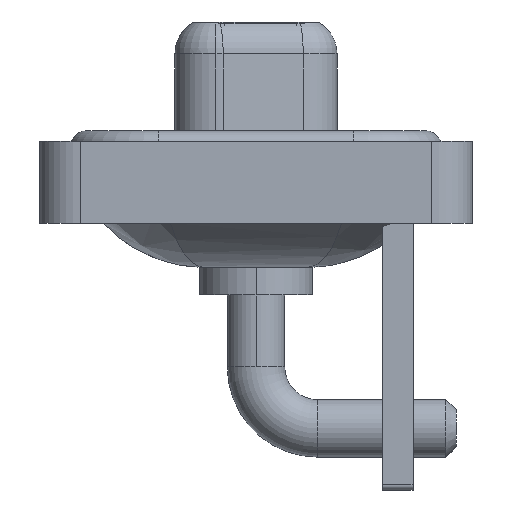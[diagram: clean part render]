
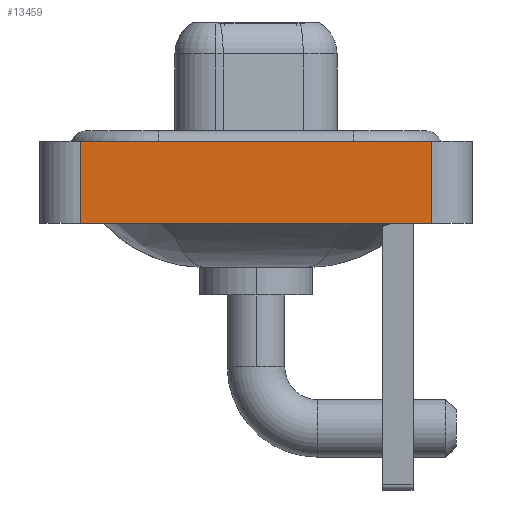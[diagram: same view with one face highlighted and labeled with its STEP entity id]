
A CAD part, left-side view. The second image highlights one B-rep face of the part: STEP entity #13459.
In plain terms, the highlighted planar face has unit normal (-1, 0, 0).
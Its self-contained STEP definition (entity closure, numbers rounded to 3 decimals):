
#3 = ORIENTED_EDGE ( 'NONE', *, *, #13370, .F. ) ;
#154 = ORIENTED_EDGE ( 'NONE', *, *, #11582, .T. ) ;
#654 = VERTEX_POINT ( 'NONE', #11953 ) ;
#843 = EDGE_LOOP ( 'NONE', ( #16155, #3, #2913, #154 ) ) ;
#848 = VERTEX_POINT ( 'NONE', #10019 ) ;
#1417 = DIRECTION ( 'NONE',  ( 0., -1., 0. ) ) ;
#1801 = VECTOR ( 'NONE', #1417, 1000. ) ;
#1831 = FACE_OUTER_BOUND ( 'NONE', #843, .T. ) ;
#2157 = CARTESIAN_POINT ( 'NONE',  ( -7.25, -8.55, 0.4 ) ) ;
#2572 = LINE ( 'NONE', #13953, #7736 ) ;
#2913 = ORIENTED_EDGE ( 'NONE', *, *, #6395, .F. ) ;
#3196 = DIRECTION ( 'NONE',  ( 0., 0., 1. ) ) ;
#4407 = VERTEX_POINT ( 'NONE', #2157 ) ;
#4519 = LINE ( 'NONE', #12037, #7982 ) ;
#5440 = PLANE ( 'NONE',  #14639 ) ;
#5573 = CARTESIAN_POINT ( 'NONE',  ( -7.25, -8.55, -3.6 ) ) ;
#6395 = EDGE_CURVE ( 'NONE', #848, #654, #15931, .T. ) ;
#6702 = DIRECTION ( 'NONE',  ( 0., 0., 1. ) ) ;
#6780 = DIRECTION ( 'NONE',  ( 0., 0., 1. ) ) ;
#7736 = VECTOR ( 'NONE', #9082, 1000. ) ;
#7982 = VECTOR ( 'NONE', #6702, 1000. ) ;
#8020 = CARTESIAN_POINT ( 'NONE',  ( -7.25, -8.55, -3.6 ) ) ;
#8755 = VECTOR ( 'NONE', #3196, 1000. ) ;
#8906 = VERTEX_POINT ( 'NONE', #5573 ) ;
#9082 = DIRECTION ( 'NONE',  ( 0., -1., 0. ) ) ;
#9191 = DIRECTION ( 'NONE',  ( -1., 0., 0. ) ) ;
#9547 = CARTESIAN_POINT ( 'NONE',  ( -7.25, 8.55, -3.6 ) ) ;
#10019 = CARTESIAN_POINT ( 'NONE',  ( -7.25, 8.55, -3.6 ) ) ;
#10379 = LINE ( 'NONE', #16417, #1801 ) ;
#11582 = EDGE_CURVE ( 'NONE', #848, #8906, #2572, .T. ) ;
#11953 = CARTESIAN_POINT ( 'NONE',  ( -7.25, 8.55, 0.4 ) ) ;
#12037 = CARTESIAN_POINT ( 'NONE',  ( -7.25, -8.55, -3.6 ) ) ;
#13370 = EDGE_CURVE ( 'NONE', #654, #4407, #10379, .T. ) ;
#13459 = ADVANCED_FACE ( 'NONE', ( #1831 ), #5440, .T. ) ;
#13953 = CARTESIAN_POINT ( 'NONE',  ( -7.25, -8.55, -3.6 ) ) ;
#14639 = AXIS2_PLACEMENT_3D ( 'NONE', #8020, #9191, #6780 ) ;
#15319 = EDGE_CURVE ( 'NONE', #8906, #4407, #4519, .T. ) ;
#15931 = LINE ( 'NONE', #9547, #8755 ) ;
#16155 = ORIENTED_EDGE ( 'NONE', *, *, #15319, .T. ) ;
#16417 = CARTESIAN_POINT ( 'NONE',  ( -7.25, -8.55, 0.4 ) ) ;
